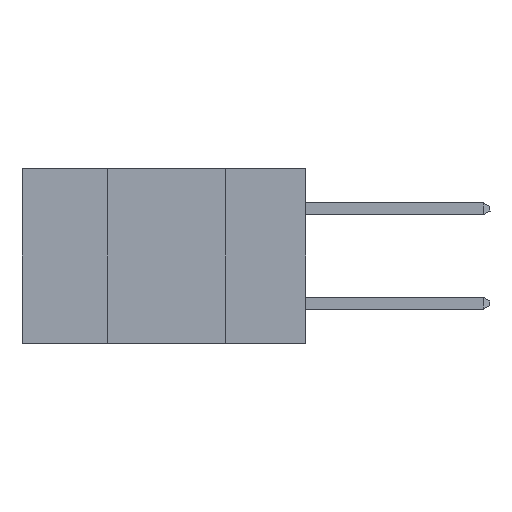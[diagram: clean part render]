
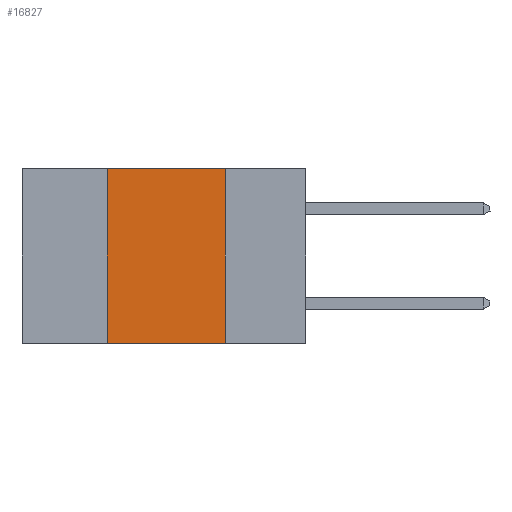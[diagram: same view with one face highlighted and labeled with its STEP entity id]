
A CAD part, left-side view. The second image highlights one B-rep face of the part: STEP entity #16827.
In plain terms, the highlighted planar face has unit normal (-1, 0, 0).
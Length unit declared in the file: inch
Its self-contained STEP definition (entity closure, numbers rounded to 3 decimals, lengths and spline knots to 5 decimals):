
#408 = ORIENTED_EDGE ( 'NONE', *, *, #22879, .F. ) ;
#446 = CARTESIAN_POINT ( 'NONE',  ( 0., 0.6, -0.37 ) ) ;
#2604 = VERTEX_POINT ( 'NONE', #20840 ) ;
#3574 = CARTESIAN_POINT ( 'NONE',  ( 0., 0.42, 0. ) ) ;
#5358 = DIRECTION ( 'NONE',  ( 0., -1., 0. ) ) ;
#6381 = CARTESIAN_POINT ( 'NONE',  ( 0., 0.42, 0. ) ) ;
#6785 = VERTEX_POINT ( 'NONE', #8768 ) ;
#7296 = LINE ( 'NONE', #446, #27256 ) ;
#7359 = EDGE_LOOP ( 'NONE', ( #408, #28436, #12174, #28764 ) ) ;
#8220 = EDGE_CURVE ( 'NONE', #20615, #2604, #14343, .T. ) ;
#8768 = CARTESIAN_POINT ( 'NONE',  ( 0., 0.17, -0.37 ) ) ;
#11160 = DIRECTION ( 'NONE',  ( 0., -1., 0. ) ) ;
#11537 = EDGE_CURVE ( 'NONE', #21630, #20615, #14186, .T. ) ;
#12174 = ORIENTED_EDGE ( 'NONE', *, *, #11537, .F. ) ;
#12673 = DIRECTION ( 'NONE',  ( 0., 0., -1. ) ) ;
#12968 = EDGE_CURVE ( 'NONE', #21630, #6785, #7296, .T. ) ;
#13770 = DIRECTION ( 'NONE',  ( 1., 0., 0. ) ) ;
#13972 = PLANE ( 'NONE',  #16455 ) ;
#14186 = LINE ( 'NONE', #6381, #24153 ) ;
#14343 = LINE ( 'NONE', #15939, #26440 ) ;
#15939 = CARTESIAN_POINT ( 'NONE',  ( 0., 0.6, 0. ) ) ;
#16455 = AXIS2_PLACEMENT_3D ( 'NONE', #20833, #13770, #20541 ) ;
#16827 = ADVANCED_FACE ( 'NONE', ( #23881 ), #13972, .F. ) ;
#20541 = DIRECTION ( 'NONE',  ( 0., 0., -1. ) ) ;
#20615 = VERTEX_POINT ( 'NONE', #3574 ) ;
#20734 = DIRECTION ( 'NONE',  ( 0., 0., 1. ) ) ;
#20833 = CARTESIAN_POINT ( 'NONE',  ( 0., 0.6, 0. ) ) ;
#20840 = CARTESIAN_POINT ( 'NONE',  ( 0., 0.17, 0. ) ) ;
#21630 = VERTEX_POINT ( 'NONE', #22132 ) ;
#22132 = CARTESIAN_POINT ( 'NONE',  ( 0., 0.42, -0.37 ) ) ;
#22879 = EDGE_CURVE ( 'NONE', #2604, #6785, #25102, .T. ) ;
#22974 = VECTOR ( 'NONE', #12673, 39.37008 ) ;
#23881 = FACE_OUTER_BOUND ( 'NONE', #7359, .T. ) ;
#24153 = VECTOR ( 'NONE', #20734, 39.37008 ) ;
#24203 = CARTESIAN_POINT ( 'NONE',  ( 0., 0.17, 0. ) ) ;
#25102 = LINE ( 'NONE', #24203, #22974 ) ;
#26440 = VECTOR ( 'NONE', #11160, 39.37008 ) ;
#27256 = VECTOR ( 'NONE', #5358, 39.37008 ) ;
#28436 = ORIENTED_EDGE ( 'NONE', *, *, #8220, .F. ) ;
#28764 = ORIENTED_EDGE ( 'NONE', *, *, #12968, .T. ) ;
